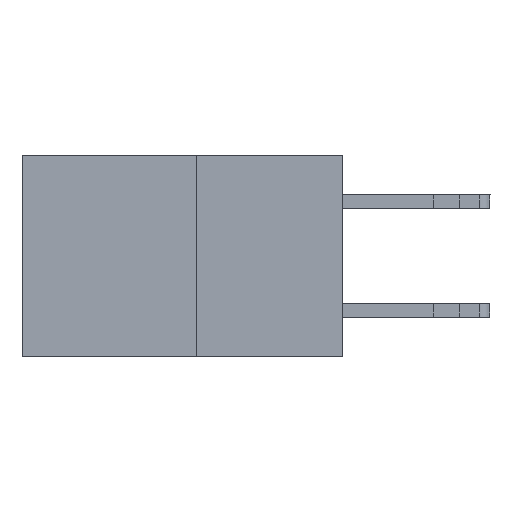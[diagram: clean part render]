
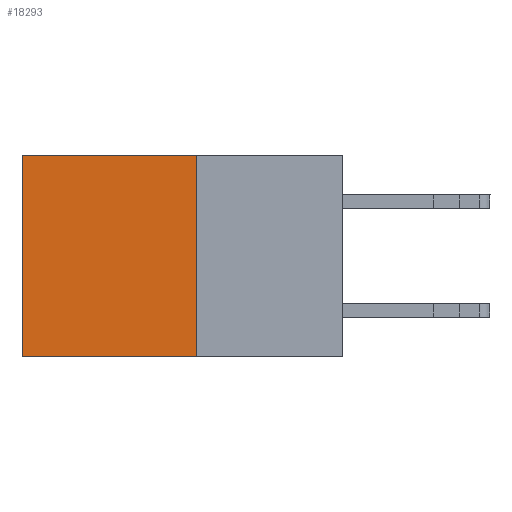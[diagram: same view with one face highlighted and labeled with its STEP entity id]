
A CAD part, left-side view. The second image highlights one B-rep face of the part: STEP entity #18293.
In plain terms, the highlighted planar face has unit normal (-1, 0, 0).
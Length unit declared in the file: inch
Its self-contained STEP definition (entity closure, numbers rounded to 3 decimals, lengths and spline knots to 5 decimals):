
#60 = VERTEX_POINT ( 'NONE', #10407 ) ;
#211 = CARTESIAN_POINT ( 'NONE',  ( 0.277, 0.27, -0.37 ) ) ;
#599 = EDGE_LOOP ( 'NONE', ( #15710, #14768, #4444, #7078 ) ) ;
#637 = EDGE_CURVE ( 'NONE', #9184, #60, #6366, .T. ) ;
#1964 = CARTESIAN_POINT ( 'NONE',  ( 0.277, 0.27, -0.37 ) ) ;
#2479 = CARTESIAN_POINT ( 'NONE',  ( 0.277, 0.59, 0. ) ) ;
#2622 = LINE ( 'NONE', #12222, #14752 ) ;
#2699 = DIRECTION ( 'NONE',  ( 0., 0., -1. ) ) ;
#3104 = VECTOR ( 'NONE', #7368, 39.37008 ) ;
#4444 = ORIENTED_EDGE ( 'NONE', *, *, #19377, .F. ) ;
#4509 = DIRECTION ( 'NONE',  ( 0., 0., -1. ) ) ;
#4639 = VECTOR ( 'NONE', #2699, 39.37008 ) ;
#5679 = CARTESIAN_POINT ( 'NONE',  ( 0.277, 0.27, 0. ) ) ;
#6130 = VERTEX_POINT ( 'NONE', #2479 ) ;
#6366 = LINE ( 'NONE', #12797, #10470 ) ;
#7078 = ORIENTED_EDGE ( 'NONE', *, *, #7533, .T. ) ;
#7368 = DIRECTION ( 'NONE',  ( 0., 1., 0. ) ) ;
#7440 = LINE ( 'NONE', #13985, #4639 ) ;
#7533 = EDGE_CURVE ( 'NONE', #12969, #6130, #18340, .T. ) ;
#7662 = AXIS2_PLACEMENT_3D ( 'NONE', #1964, #8496, #9969 ) ;
#8496 = DIRECTION ( 'NONE',  ( 1., 0., 0. ) ) ;
#9184 = VERTEX_POINT ( 'NONE', #211 ) ;
#9969 = DIRECTION ( 'NONE',  ( 0., 0., -1. ) ) ;
#10407 = CARTESIAN_POINT ( 'NONE',  ( 0.277, 0.59, -0.37 ) ) ;
#10470 = VECTOR ( 'NONE', #19128, 39.37008 ) ;
#11757 = EDGE_CURVE ( 'NONE', #6130, #60, #7440, .T. ) ;
#12222 = CARTESIAN_POINT ( 'NONE',  ( 0.277, 0.27, -0.37 ) ) ;
#12797 = CARTESIAN_POINT ( 'NONE',  ( 0.277, 0.27, -0.37 ) ) ;
#12969 = VERTEX_POINT ( 'NONE', #19814 ) ;
#13985 = CARTESIAN_POINT ( 'NONE',  ( 0.277, 0.59, -0.37 ) ) ;
#14752 = VECTOR ( 'NONE', #4509, 39.37008 ) ;
#14768 = ORIENTED_EDGE ( 'NONE', *, *, #637, .F. ) ;
#15140 = FACE_OUTER_BOUND ( 'NONE', #599, .T. ) ;
#15710 = ORIENTED_EDGE ( 'NONE', *, *, #11757, .T. ) ;
#17994 = PLANE ( 'NONE',  #7662 ) ;
#18293 = ADVANCED_FACE ( 'NONE', ( #15140 ), #17994, .F. ) ;
#18340 = LINE ( 'NONE', #5679, #3104 ) ;
#19128 = DIRECTION ( 'NONE',  ( 0., 1., 0. ) ) ;
#19377 = EDGE_CURVE ( 'NONE', #12969, #9184, #2622, .T. ) ;
#19814 = CARTESIAN_POINT ( 'NONE',  ( 0.277, 0.27, 0. ) ) ;
